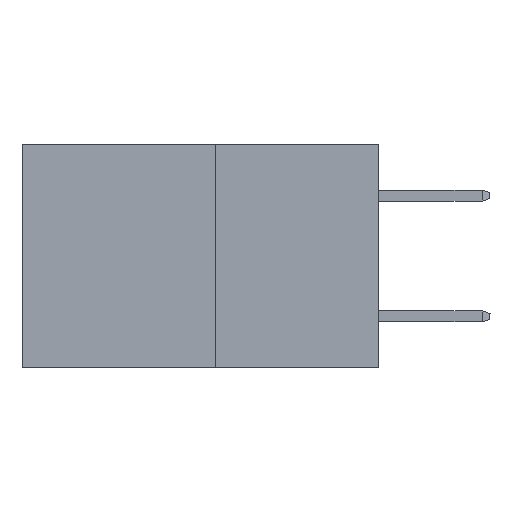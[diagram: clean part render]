
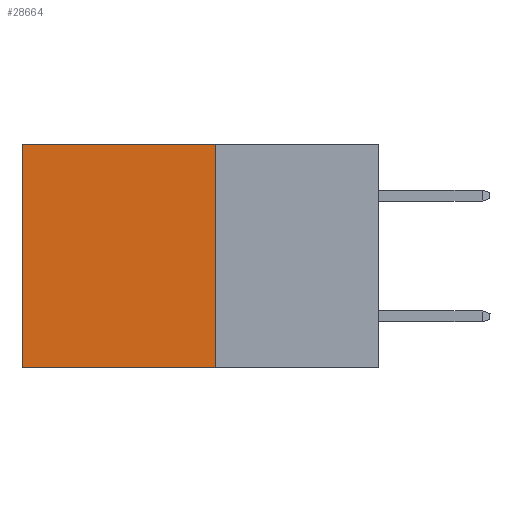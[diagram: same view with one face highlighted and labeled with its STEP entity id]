
A CAD part, left-side view. The second image highlights one B-rep face of the part: STEP entity #28664.
In plain terms, the highlighted planar face has unit normal (-1, 0, 0).
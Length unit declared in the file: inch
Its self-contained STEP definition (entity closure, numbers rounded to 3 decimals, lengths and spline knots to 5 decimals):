
#1800 = CARTESIAN_POINT ( 'NONE',  ( 0.277, 0.59, -0.37 ) ) ;
#2006 = EDGE_LOOP ( 'NONE', ( #9697, #25894, #21532, #20612 ) ) ;
#2404 = FACE_OUTER_BOUND ( 'NONE', #2006, .T. ) ;
#3672 = EDGE_CURVE ( 'NONE', #19727, #6943, #29320, .T. ) ;
#4769 = VECTOR ( 'NONE', #6767, 39.37008 ) ;
#6767 = DIRECTION ( 'NONE',  ( 0., 1., 0. ) ) ;
#6943 = VERTEX_POINT ( 'NONE', #20160 ) ;
#8455 = LINE ( 'NONE', #28259, #14868 ) ;
#9697 = ORIENTED_EDGE ( 'NONE', *, *, #24820, .T. ) ;
#10704 = CARTESIAN_POINT ( 'NONE',  ( 0.277, 0.27, -0.37 ) ) ;
#10817 = DIRECTION ( 'NONE',  ( 0., 0., -1. ) ) ;
#11168 = LINE ( 'NONE', #23130, #4769 ) ;
#11296 = VERTEX_POINT ( 'NONE', #15968 ) ;
#14099 = EDGE_CURVE ( 'NONE', #6943, #32693, #11168, .T. ) ;
#14549 = CARTESIAN_POINT ( 'NONE',  ( 0.277, 0.59, -0.37 ) ) ;
#14565 = PLANE ( 'NONE',  #31135 ) ;
#14621 = DIRECTION ( 'NONE',  ( 0., 1., 0. ) ) ;
#14868 = VECTOR ( 'NONE', #14621, 39.37008 ) ;
#15641 = VECTOR ( 'NONE', #10817, 39.37008 ) ;
#15968 = CARTESIAN_POINT ( 'NONE',  ( 0.277, 0.59, 0. ) ) ;
#17288 = DIRECTION ( 'NONE',  ( 0., 0., -1. ) ) ;
#19727 = VERTEX_POINT ( 'NONE', #30876 ) ;
#20160 = CARTESIAN_POINT ( 'NONE',  ( 0.277, 0.27, -0.37 ) ) ;
#20612 = ORIENTED_EDGE ( 'NONE', *, *, #22499, .T. ) ;
#21532 = ORIENTED_EDGE ( 'NONE', *, *, #3672, .F. ) ;
#22499 = EDGE_CURVE ( 'NONE', #19727, #11296, #8455, .T. ) ;
#23130 = CARTESIAN_POINT ( 'NONE',  ( 0.277, 0.27, -0.37 ) ) ;
#24820 = EDGE_CURVE ( 'NONE', #11296, #32693, #32977, .T. ) ;
#25706 = VECTOR ( 'NONE', #28305, 39.37008 ) ;
#25894 = ORIENTED_EDGE ( 'NONE', *, *, #14099, .F. ) ;
#28259 = CARTESIAN_POINT ( 'NONE',  ( 0.277, 0.27, 0. ) ) ;
#28305 = DIRECTION ( 'NONE',  ( 0., 0., -1. ) ) ;
#28664 = ADVANCED_FACE ( 'NONE', ( #2404 ), #14565, .F. ) ;
#29320 = LINE ( 'NONE', #10704, #15641 ) ;
#30876 = CARTESIAN_POINT ( 'NONE',  ( 0.277, 0.27, 0. ) ) ;
#30922 = CARTESIAN_POINT ( 'NONE',  ( 0.277, 0.27, -0.37 ) ) ;
#31135 = AXIS2_PLACEMENT_3D ( 'NONE', #30922, #33673, #17288 ) ;
#32693 = VERTEX_POINT ( 'NONE', #1800 ) ;
#32977 = LINE ( 'NONE', #14549, #25706 ) ;
#33673 = DIRECTION ( 'NONE',  ( 1., 0., 0. ) ) ;
